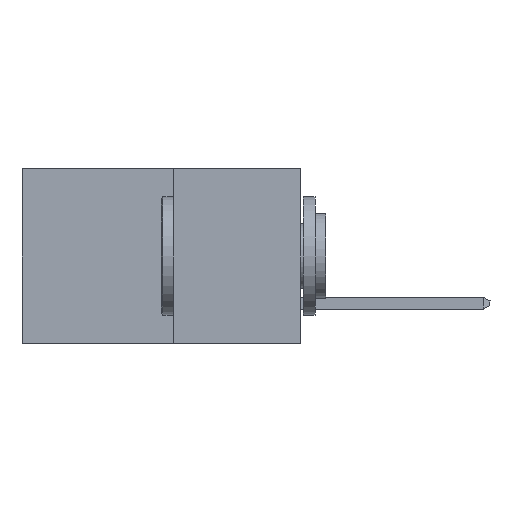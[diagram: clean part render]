
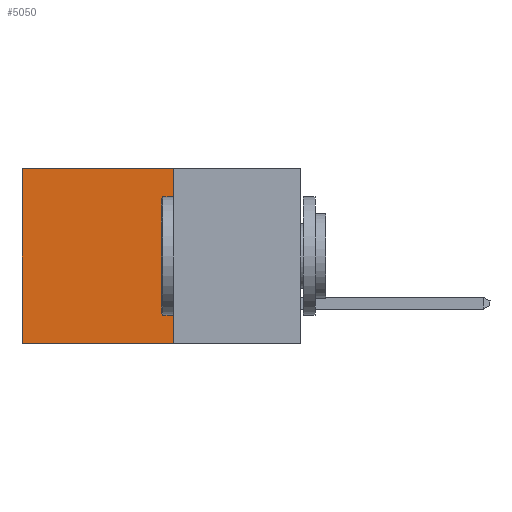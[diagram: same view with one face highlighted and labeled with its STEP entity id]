
A CAD part, left-side view. The second image highlights one B-rep face of the part: STEP entity #5050.
In plain terms, the highlighted planar face has unit normal (-1, 0, 0).
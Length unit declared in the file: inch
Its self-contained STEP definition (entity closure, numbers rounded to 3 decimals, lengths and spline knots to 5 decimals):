
#1007 = ORIENTED_EDGE ( 'NONE', *, *, #10135, .T. ) ;
#1035 = CARTESIAN_POINT ( 'NONE',  ( 0.277, 0.59, -0.37 ) ) ;
#1550 = LINE ( 'NONE', #10433, #3649 ) ;
#3391 = ORIENTED_EDGE ( 'NONE', *, *, #5307, .F. ) ;
#3623 = VERTEX_POINT ( 'NONE', #10456 ) ;
#3649 = VECTOR ( 'NONE', #6285, 39.37008 ) ;
#4119 = FACE_OUTER_BOUND ( 'NONE', #5186, .T. ) ;
#4231 = DIRECTION ( 'NONE',  ( 0., 1., 0. ) ) ;
#4251 = CARTESIAN_POINT ( 'NONE',  ( 0.277, 0.27, -0.37 ) ) ;
#4429 = LINE ( 'NONE', #1035, #6491 ) ;
#5010 = VERTEX_POINT ( 'NONE', #6186 ) ;
#5050 = ADVANCED_FACE ( 'NONE', ( #4119 ), #5823, .F. ) ;
#5116 = VERTEX_POINT ( 'NONE', #5345 ) ;
#5186 = EDGE_LOOP ( 'NONE', ( #1007, #3391, #5821, #8064 ) ) ;
#5307 = EDGE_CURVE ( 'NONE', #3623, #5010, #6081, .T. ) ;
#5345 = CARTESIAN_POINT ( 'NONE',  ( 0.277, 0.59, 0. ) ) ;
#5501 = DIRECTION ( 'NONE',  ( 0., 1., 0. ) ) ;
#5627 = LINE ( 'NONE', #8851, #7643 ) ;
#5735 = DIRECTION ( 'NONE',  ( 0., 0., -1. ) ) ;
#5747 = DIRECTION ( 'NONE',  ( 1., 0., 0. ) ) ;
#5821 = ORIENTED_EDGE ( 'NONE', *, *, #10823, .F. ) ;
#5823 = PLANE ( 'NONE',  #9953 ) ;
#5956 = CARTESIAN_POINT ( 'NONE',  ( 0.277, 0.27, -0.37 ) ) ;
#6081 = LINE ( 'NONE', #4251, #8300 ) ;
#6186 = CARTESIAN_POINT ( 'NONE',  ( 0.277, 0.59, -0.37 ) ) ;
#6285 = DIRECTION ( 'NONE',  ( 0., 0., -1. ) ) ;
#6422 = DIRECTION ( 'NONE',  ( 0., 0., -1. ) ) ;
#6491 = VECTOR ( 'NONE', #6422, 39.37008 ) ;
#7643 = VECTOR ( 'NONE', #5501, 39.37008 ) ;
#7786 = EDGE_CURVE ( 'NONE', #7917, #5116, #5627, .T. ) ;
#7917 = VERTEX_POINT ( 'NONE', #8150 ) ;
#8064 = ORIENTED_EDGE ( 'NONE', *, *, #7786, .T. ) ;
#8150 = CARTESIAN_POINT ( 'NONE',  ( 0.277, 0.27, 0. ) ) ;
#8300 = VECTOR ( 'NONE', #4231, 39.37008 ) ;
#8851 = CARTESIAN_POINT ( 'NONE',  ( 0.277, 0.27, 0. ) ) ;
#9953 = AXIS2_PLACEMENT_3D ( 'NONE', #5956, #5747, #5735 ) ;
#10135 = EDGE_CURVE ( 'NONE', #5116, #5010, #4429, .T. ) ;
#10433 = CARTESIAN_POINT ( 'NONE',  ( 0.277, 0.27, -0.37 ) ) ;
#10456 = CARTESIAN_POINT ( 'NONE',  ( 0.277, 0.27, -0.37 ) ) ;
#10823 = EDGE_CURVE ( 'NONE', #7917, #3623, #1550, .T. ) ;
